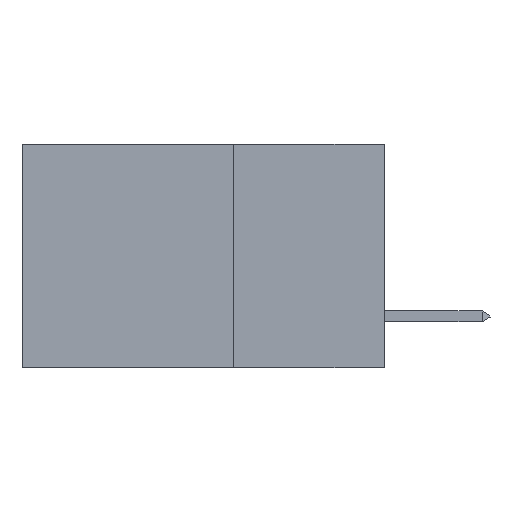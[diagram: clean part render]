
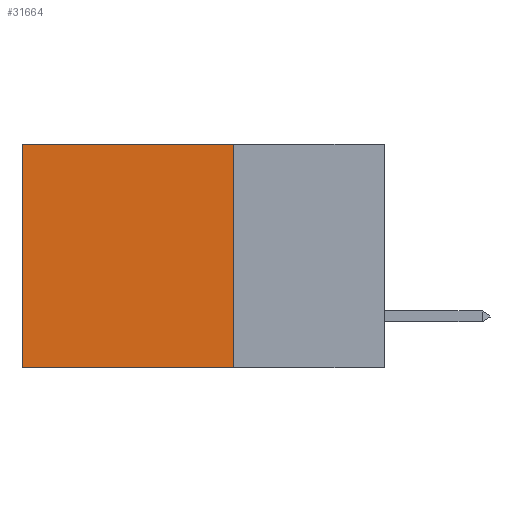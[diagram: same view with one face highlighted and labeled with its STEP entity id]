
A CAD part, left-side view. The second image highlights one B-rep face of the part: STEP entity #31664.
In plain terms, the highlighted planar face has unit normal (-1, 0, 0).
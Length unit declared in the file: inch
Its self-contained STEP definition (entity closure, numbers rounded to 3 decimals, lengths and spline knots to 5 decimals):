
#22 = FACE_OUTER_BOUND ( 'NONE', #2799, .T. ) ;
#26 = VECTOR ( 'NONE', #22969, 39.37008 ) ;
#1397 = CARTESIAN_POINT ( 'NONE',  ( 0.2875, 0.25, -0.37 ) ) ;
#2384 = LINE ( 'NONE', #14852, #25027 ) ;
#2799 = EDGE_LOOP ( 'NONE', ( #19410, #5763, #24311, #8717 ) ) ;
#4419 = PLANE ( 'NONE',  #26847 ) ;
#4932 = LINE ( 'NONE', #6855, #24530 ) ;
#5391 = DIRECTION ( 'NONE',  ( 1., 0., 0. ) ) ;
#5763 = ORIENTED_EDGE ( 'NONE', *, *, #24788, .F. ) ;
#6855 = CARTESIAN_POINT ( 'NONE',  ( 0.2875, 0.25, 0. ) ) ;
#7270 = DIRECTION ( 'NONE',  ( 0., 0., -1. ) ) ;
#7950 = VERTEX_POINT ( 'NONE', #10051 ) ;
#8717 = ORIENTED_EDGE ( 'NONE', *, *, #14485, .T. ) ;
#10051 = CARTESIAN_POINT ( 'NONE',  ( 0.2875, 0.25, -0.37 ) ) ;
#10591 = VECTOR ( 'NONE', #17735, 39.37008 ) ;
#11997 = EDGE_CURVE ( 'NONE', #15656, #20645, #2384, .T. ) ;
#14485 = EDGE_CURVE ( 'NONE', #32410, #15656, #22262, .T. ) ;
#14852 = CARTESIAN_POINT ( 'NONE',  ( 0.2875, 0.6, 0. ) ) ;
#15656 = VERTEX_POINT ( 'NONE', #31364 ) ;
#17735 = DIRECTION ( 'NONE',  ( 0., 1., 0. ) ) ;
#19410 = ORIENTED_EDGE ( 'NONE', *, *, #11997, .T. ) ;
#20645 = VERTEX_POINT ( 'NONE', #21376 ) ;
#21376 = CARTESIAN_POINT ( 'NONE',  ( 0.2875, 0.6, -0.37 ) ) ;
#22262 = LINE ( 'NONE', #25745, #26 ) ;
#22969 = DIRECTION ( 'NONE',  ( 0., 1., 0. ) ) ;
#24311 = ORIENTED_EDGE ( 'NONE', *, *, #30320, .F. ) ;
#24530 = VECTOR ( 'NONE', #31398, 39.37008 ) ;
#24735 = DIRECTION ( 'NONE',  ( 0., 0., -1. ) ) ;
#24788 = EDGE_CURVE ( 'NONE', #7950, #20645, #25373, .T. ) ;
#25027 = VECTOR ( 'NONE', #7270, 39.37008 ) ;
#25373 = LINE ( 'NONE', #1397, #10591 ) ;
#25745 = CARTESIAN_POINT ( 'NONE',  ( 0.2875, 0.25, 0. ) ) ;
#26847 = AXIS2_PLACEMENT_3D ( 'NONE', #35473, #5391, #24735 ) ;
#30320 = EDGE_CURVE ( 'NONE', #32410, #7950, #4932, .T. ) ;
#30466 = CARTESIAN_POINT ( 'NONE',  ( 0.2875, 0.25, 0. ) ) ;
#31364 = CARTESIAN_POINT ( 'NONE',  ( 0.2875, 0.6, 0. ) ) ;
#31398 = DIRECTION ( 'NONE',  ( 0., 0., -1. ) ) ;
#31664 = ADVANCED_FACE ( 'NONE', ( #22 ), #4419, .F. ) ;
#32410 = VERTEX_POINT ( 'NONE', #30466 ) ;
#35473 = CARTESIAN_POINT ( 'NONE',  ( 0.2875, 0.25, 0. ) ) ;
